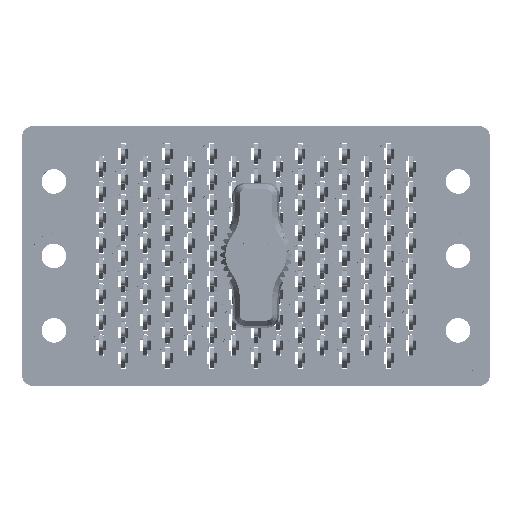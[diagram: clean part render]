
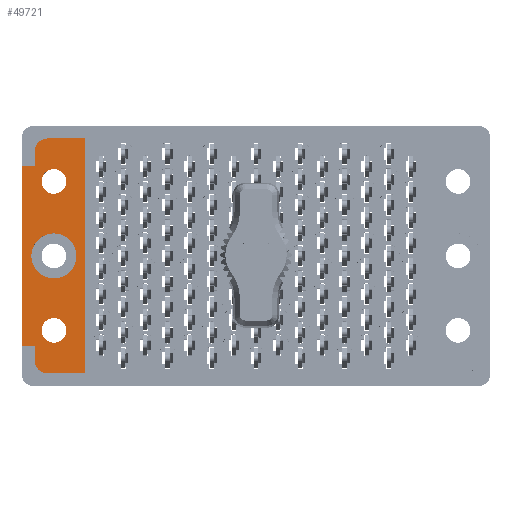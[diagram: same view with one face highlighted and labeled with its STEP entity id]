
A CAD part, top view. The second image highlights one B-rep face of the part: STEP entity #49721.
In plain terms, the highlighted planar face has unit normal (0, 0, 1).
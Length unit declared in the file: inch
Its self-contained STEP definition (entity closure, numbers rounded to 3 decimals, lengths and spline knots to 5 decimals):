
#6 = DIRECTION ( 'NONE',  ( 0., 0., 1. ) ) ;
#430 = CIRCLE ( 'NONE', #3580, 0.0725 ) ;
#512 = EDGE_CURVE ( 'NONE', #19142, #79244, #52107, .T. ) ;
#2185 = DIRECTION ( 'NONE',  ( 1., 0., 0. ) ) ;
#2530 = CARTESIAN_POINT ( 'NONE',  ( -1.3, 0.615, -0.117 ) ) ;
#3183 = FACE_BOUND ( 'NONE', #46580, .T. ) ;
#3580 = AXIS2_PLACEMENT_3D ( 'NONE', #54600, #20608, #5039 ) ;
#4056 = CARTESIAN_POINT ( 'NONE',  ( -1.225, -0.69, -0.117 ) ) ;
#5039 = DIRECTION ( 'NONE',  ( 1., 0., 0. ) ) ;
#5784 = PLANE ( 'NONE',  #89531 ) ;
#6188 = VECTOR ( 'NONE', #30086, 39.37008 ) ;
#6705 = DIRECTION ( 'NONE',  ( 0., 0., 1. ) ) ;
#7628 = ORIENTED_EDGE ( 'NONE', *, *, #49117, .F. ) ;
#7873 = CIRCLE ( 'NONE', #35845, 0.0725 ) ;
#9577 = AXIS2_PLACEMENT_3D ( 'NONE', #44346, #93471, #102140 ) ;
#10429 = LINE ( 'NONE', #68412, #94445 ) ;
#11674 = EDGE_CURVE ( 'NONE', #32640, #26775, #79077, .T. ) ;
#14378 = ORIENTED_EDGE ( 'NONE', *, *, #83425, .T. ) ;
#14900 = VERTEX_POINT ( 'NONE', #84946 ) ;
#15553 = CIRCLE ( 'NONE', #44789, 0.0725 ) ;
#16899 = EDGE_CURVE ( 'NONE', #19142, #37109, #102980, .T. ) ;
#18435 = DIRECTION ( 'NONE',  ( 0., 0., 1. ) ) ;
#19142 = VERTEX_POINT ( 'NONE', #64831 ) ;
#20608 = DIRECTION ( 'NONE',  ( 0., 0., 1. ) ) ;
#21380 = CARTESIAN_POINT ( 'NONE',  ( -1.005, 0.7625, -0.117 ) ) ;
#25163 = EDGE_CURVE ( 'NONE', #68887, #94000, #7873, .T. ) ;
#25347 = DIRECTION ( 'NONE',  ( 1., 0., 0. ) ) ;
#25398 = CARTESIAN_POINT ( 'NONE',  ( -1.1875, 0.4375, -0.117 ) ) ;
#26775 = VERTEX_POINT ( 'NONE', #4056 ) ;
#26779 = CARTESIAN_POINT ( 'NONE',  ( -1.1875, -0.4375, -0.117 ) ) ;
#27199 = ORIENTED_EDGE ( 'NONE', *, *, #100649, .T. ) ;
#27299 = CIRCLE ( 'NONE', #83422, 0.1325 ) ;
#27358 = DIRECTION ( 'NONE',  ( -1., 0., 0. ) ) ;
#27832 = DIRECTION ( 'NONE',  ( 0., 0., 1. ) ) ;
#28888 = CARTESIAN_POINT ( 'NONE',  ( -1.375, -0.7625, -0.117 ) ) ;
#29681 = ORIENTED_EDGE ( 'NONE', *, *, #52386, .F. ) ;
#29917 = DIRECTION ( 'NONE',  ( 0., -1., 0. ) ) ;
#30086 = DIRECTION ( 'NONE',  ( -1., 0., 0. ) ) ;
#30494 = CARTESIAN_POINT ( 'NONE',  ( -1.005, -0.69, -0.117 ) ) ;
#30716 = VERTEX_POINT ( 'NONE', #83456 ) ;
#30828 = CIRCLE ( 'NONE', #35944, 0.075 ) ;
#31643 = CARTESIAN_POINT ( 'NONE',  ( -1.375, -0.5285, -0.117 ) ) ;
#32640 = VERTEX_POINT ( 'NONE', #30494 ) ;
#33994 = ORIENTED_EDGE ( 'NONE', *, *, #54303, .T. ) ;
#35845 = AXIS2_PLACEMENT_3D ( 'NONE', #26779, #18435, #2185 ) ;
#35944 = AXIS2_PLACEMENT_3D ( 'NONE', #84934, #27832, #51718 ) ;
#37109 = VERTEX_POINT ( 'NONE', #64390 ) ;
#37524 = CARTESIAN_POINT ( 'NONE',  ( -1.3, 0., -0.117 ) ) ;
#39407 = FACE_BOUND ( 'NONE', #92219, .T. ) ;
#41417 = EDGE_CURVE ( 'NONE', #32640, #83828, #54485, .T. ) ;
#41491 = VERTEX_POINT ( 'NONE', #62587 ) ;
#41650 = VECTOR ( 'NONE', #88370, 39.37008 ) ;
#43715 = DIRECTION ( 'NONE',  ( 1., 0., 0. ) ) ;
#44346 = CARTESIAN_POINT ( 'NONE',  ( -1.225, -0.615, -0.117 ) ) ;
#44689 = CARTESIAN_POINT ( 'NONE',  ( 0., -0.5285, -0.117 ) ) ;
#44789 = AXIS2_PLACEMENT_3D ( 'NONE', #98460, #6705, #98104 ) ;
#44831 = DIRECTION ( 'NONE',  ( 0., 0., 1. ) ) ;
#45283 = VERTEX_POINT ( 'NONE', #2530 ) ;
#45817 = FACE_BOUND ( 'NONE', #89993, .T. ) ;
#45958 = EDGE_CURVE ( 'NONE', #37109, #26775, #100787, .T. ) ;
#46580 = EDGE_LOOP ( 'NONE', ( #7628, #67477 ) ) ;
#47478 = VECTOR ( 'NONE', #76383, 39.37008 ) ;
#47533 = ORIENTED_EDGE ( 'NONE', *, *, #512, .F. ) ;
#48572 = DIRECTION ( 'NONE',  ( 0., 0., 1. ) ) ;
#48909 = CARTESIAN_POINT ( 'NONE',  ( -1.3, 0., -0.117 ) ) ;
#49117 = EDGE_CURVE ( 'NONE', #83135, #14900, #53760, .T. ) ;
#49721 = ADVANCED_FACE ( 'NONE', ( #45817, #39407, #3183, #67834 ), #5784, .T. ) ;
#51326 = LINE ( 'NONE', #60530, #47478 ) ;
#51718 = DIRECTION ( 'NONE',  ( 1., 0., 0. ) ) ;
#52107 = LINE ( 'NONE', #44689, #102475 ) ;
#52353 = CARTESIAN_POINT ( 'NONE',  ( -1.375, 0.5285, -0.117 ) ) ;
#52386 = EDGE_CURVE ( 'NONE', #72593, #30716, #15553, .T. ) ;
#53760 = CIRCLE ( 'NONE', #66609, 0.1325 ) ;
#54303 = EDGE_CURVE ( 'NONE', #41491, #45283, #30828, .T. ) ;
#54485 = LINE ( 'NONE', #21380, #94470 ) ;
#54600 = CARTESIAN_POINT ( 'NONE',  ( -1.1875, -0.4375, -0.117 ) ) ;
#60530 = CARTESIAN_POINT ( 'NONE',  ( -1.375, 0.7625, -0.117 ) ) ;
#60592 = VECTOR ( 'NONE', #97277, 39.37008 ) ;
#61096 = CIRCLE ( 'NONE', #66746, 0.0725 ) ;
#62587 = CARTESIAN_POINT ( 'NONE',  ( -1.225, 0.69, -0.117 ) ) ;
#63211 = ORIENTED_EDGE ( 'NONE', *, *, #69280, .F. ) ;
#63606 = DIRECTION ( 'NONE',  ( 1., 0., 0. ) ) ;
#64390 = CARTESIAN_POINT ( 'NONE',  ( -1.3, -0.615, -0.117 ) ) ;
#64831 = CARTESIAN_POINT ( 'NONE',  ( -1.3, -0.5285, -0.117 ) ) ;
#66185 = EDGE_CURVE ( 'NONE', #83828, #41491, #104454, .T. ) ;
#66414 = ORIENTED_EDGE ( 'NONE', *, *, #45958, .T. ) ;
#66609 = AXIS2_PLACEMENT_3D ( 'NONE', #99035, #6, #25347 ) ;
#66746 = AXIS2_PLACEMENT_3D ( 'NONE', #25398, #48572, #107041 ) ;
#67477 = ORIENTED_EDGE ( 'NONE', *, *, #97127, .F. ) ;
#67834 = FACE_OUTER_BOUND ( 'NONE', #73890, .T. ) ;
#68412 = CARTESIAN_POINT ( 'NONE',  ( 0., 0.5285, -0.117 ) ) ;
#68482 = VERTEX_POINT ( 'NONE', #95711 ) ;
#68887 = VERTEX_POINT ( 'NONE', #71657 ) ;
#69132 = DIRECTION ( 'NONE',  ( -1., 0., 0. ) ) ;
#69280 = EDGE_CURVE ( 'NONE', #94000, #68887, #430, .T. ) ;
#71233 = ORIENTED_EDGE ( 'NONE', *, *, #11674, .F. ) ;
#71323 = CARTESIAN_POINT ( 'NONE',  ( 0., 0.69, -0.117 ) ) ;
#71657 = CARTESIAN_POINT ( 'NONE',  ( -1.115, -0.4375, -0.117 ) ) ;
#72593 = VERTEX_POINT ( 'NONE', #91282 ) ;
#73890 = EDGE_LOOP ( 'NONE', ( #97230, #33994, #27199, #90282, #14378, #47533, #97423, #66414, #71233, #77511 ) ) ;
#76383 = DIRECTION ( 'NONE',  ( 0., -1., 0. ) ) ;
#77304 = DIRECTION ( 'NONE',  ( 0., 0., 1. ) ) ;
#77511 = ORIENTED_EDGE ( 'NONE', *, *, #41417, .T. ) ;
#79077 = LINE ( 'NONE', #89083, #41650 ) ;
#79244 = VERTEX_POINT ( 'NONE', #31643 ) ;
#80739 = CARTESIAN_POINT ( 'NONE',  ( -1.26, -0.4375, -0.117 ) ) ;
#82043 = CARTESIAN_POINT ( 'NONE',  ( -1.005, 0.69, -0.117 ) ) ;
#83135 = VERTEX_POINT ( 'NONE', #99184 ) ;
#83422 = AXIS2_PLACEMENT_3D ( 'NONE', #85259, #77304, #43715 ) ;
#83425 = EDGE_CURVE ( 'NONE', #84022, #79244, #51326, .T. ) ;
#83456 = CARTESIAN_POINT ( 'NONE',  ( -1.26, 0.4375, -0.117 ) ) ;
#83828 = VERTEX_POINT ( 'NONE', #82043 ) ;
#84022 = VERTEX_POINT ( 'NONE', #52353 ) ;
#84934 = CARTESIAN_POINT ( 'NONE',  ( -1.225, 0.615, -0.117 ) ) ;
#84946 = CARTESIAN_POINT ( 'NONE',  ( -1.32, 0., -0.117 ) ) ;
#85259 = CARTESIAN_POINT ( 'NONE',  ( -1.1875, 0., -0.117 ) ) ;
#86220 = ORIENTED_EDGE ( 'NONE', *, *, #25163, .F. ) ;
#86686 = ORIENTED_EDGE ( 'NONE', *, *, #105194, .F. ) ;
#87132 = DIRECTION ( 'NONE',  ( 0., 1., 0. ) ) ;
#88370 = DIRECTION ( 'NONE',  ( -1., 0., 0. ) ) ;
#89083 = CARTESIAN_POINT ( 'NONE',  ( 0., -0.69, -0.117 ) ) ;
#89531 = AXIS2_PLACEMENT_3D ( 'NONE', #28888, #44831, #63606 ) ;
#89993 = EDGE_LOOP ( 'NONE', ( #86686, #29681 ) ) ;
#90282 = ORIENTED_EDGE ( 'NONE', *, *, #96170, .T. ) ;
#91282 = CARTESIAN_POINT ( 'NONE',  ( -1.115, 0.4375, -0.117 ) ) ;
#92219 = EDGE_LOOP ( 'NONE', ( #63211, #86220 ) ) ;
#93471 = DIRECTION ( 'NONE',  ( 0., 0., 1. ) ) ;
#94000 = VERTEX_POINT ( 'NONE', #80739 ) ;
#94445 = VECTOR ( 'NONE', #69132, 39.37008 ) ;
#94470 = VECTOR ( 'NONE', #87132, 39.37008 ) ;
#95711 = CARTESIAN_POINT ( 'NONE',  ( -1.3, 0.5285, -0.117 ) ) ;
#96170 = EDGE_CURVE ( 'NONE', #68482, #84022, #10429, .T. ) ;
#97127 = EDGE_CURVE ( 'NONE', #14900, #83135, #27299, .T. ) ;
#97230 = ORIENTED_EDGE ( 'NONE', *, *, #66185, .T. ) ;
#97277 = DIRECTION ( 'NONE',  ( 0., -1., 0. ) ) ;
#97423 = ORIENTED_EDGE ( 'NONE', *, *, #16899, .T. ) ;
#97790 = VECTOR ( 'NONE', #29917, 39.37008 ) ;
#98104 = DIRECTION ( 'NONE',  ( 1., 0., 0. ) ) ;
#98460 = CARTESIAN_POINT ( 'NONE',  ( -1.1875, 0.4375, -0.117 ) ) ;
#99035 = CARTESIAN_POINT ( 'NONE',  ( -1.1875, 0., -0.117 ) ) ;
#99184 = CARTESIAN_POINT ( 'NONE',  ( -1.055, 0., -0.117 ) ) ;
#100649 = EDGE_CURVE ( 'NONE', #45283, #68482, #104464, .T. ) ;
#100787 = CIRCLE ( 'NONE', #9577, 0.075 ) ;
#102140 = DIRECTION ( 'NONE',  ( 1., 0., 0. ) ) ;
#102475 = VECTOR ( 'NONE', #27358, 39.37008 ) ;
#102980 = LINE ( 'NONE', #37524, #97790 ) ;
#104454 = LINE ( 'NONE', #71323, #6188 ) ;
#104464 = LINE ( 'NONE', #48909, #60592 ) ;
#105194 = EDGE_CURVE ( 'NONE', #30716, #72593, #61096, .T. ) ;
#107041 = DIRECTION ( 'NONE',  ( 1., 0., 0. ) ) ;
